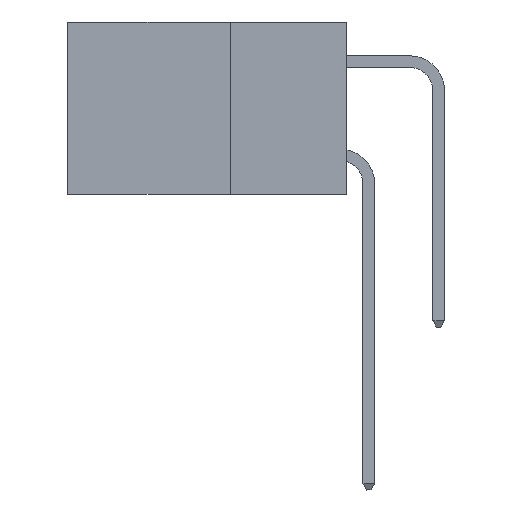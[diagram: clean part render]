
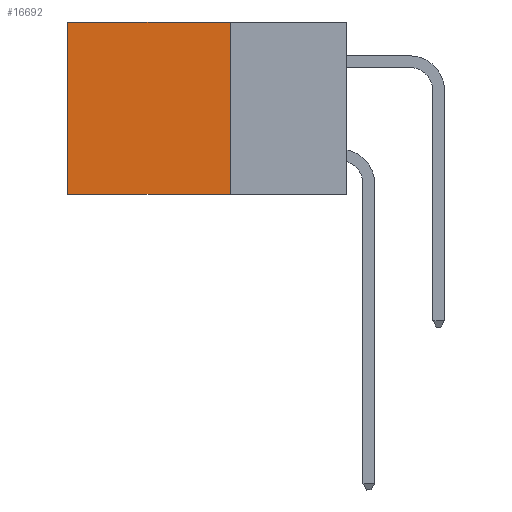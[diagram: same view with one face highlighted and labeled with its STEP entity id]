
A CAD part, left-side view. The second image highlights one B-rep face of the part: STEP entity #16692.
In plain terms, the highlighted planar face has unit normal (-1, 0, 0).
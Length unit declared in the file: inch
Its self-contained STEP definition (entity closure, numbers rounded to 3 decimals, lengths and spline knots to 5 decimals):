
#27 = LINE ( 'NONE', #17710, #20321 ) ;
#296 = DIRECTION ( 'NONE',  ( 0., 1., 0. ) ) ;
#1397 = DIRECTION ( 'NONE',  ( 1., 0., 0. ) ) ;
#1932 = DIRECTION ( 'NONE',  ( 0., 1., 0. ) ) ;
#1976 = VERTEX_POINT ( 'NONE', #5141 ) ;
#2267 = CARTESIAN_POINT ( 'NONE',  ( 0.2875, 0.6, 0. ) ) ;
#2382 = ORIENTED_EDGE ( 'NONE', *, *, #10163, .T. ) ;
#2730 = EDGE_CURVE ( 'NONE', #20494, #1976, #27, .T. ) ;
#3203 = CARTESIAN_POINT ( 'NONE',  ( 0.2875, 0.6, -0.37 ) ) ;
#3978 = EDGE_CURVE ( 'NONE', #20494, #5304, #15951, .T. ) ;
#4183 = CARTESIAN_POINT ( 'NONE',  ( 0.2875, 0.25, 0. ) ) ;
#5141 = CARTESIAN_POINT ( 'NONE',  ( 0.2875, 0.6, 0. ) ) ;
#5304 = VERTEX_POINT ( 'NONE', #8259 ) ;
#5743 = FACE_OUTER_BOUND ( 'NONE', #12007, .T. ) ;
#5843 = DIRECTION ( 'NONE',  ( 0., 0., -1. ) ) ;
#7091 = EDGE_CURVE ( 'NONE', #5304, #24852, #16056, .T. ) ;
#8259 = CARTESIAN_POINT ( 'NONE',  ( 0.2875, 0.25, -0.37 ) ) ;
#8890 = VECTOR ( 'NONE', #16130, 39.37008 ) ;
#9052 = CARTESIAN_POINT ( 'NONE',  ( 0.2875, 0.25, 0. ) ) ;
#10163 = EDGE_CURVE ( 'NONE', #1976, #24852, #10342, .T. ) ;
#10342 = LINE ( 'NONE', #2267, #18902 ) ;
#12007 = EDGE_LOOP ( 'NONE', ( #2382, #25248, #13574, #16932 ) ) ;
#12174 = CARTESIAN_POINT ( 'NONE',  ( 0.2875, 0.25, 0. ) ) ;
#13266 = VECTOR ( 'NONE', #296, 39.37008 ) ;
#13574 = ORIENTED_EDGE ( 'NONE', *, *, #3978, .F. ) ;
#15003 = AXIS2_PLACEMENT_3D ( 'NONE', #9052, #1397, #22782 ) ;
#15951 = LINE ( 'NONE', #4183, #8890 ) ;
#16056 = LINE ( 'NONE', #17455, #13266 ) ;
#16130 = DIRECTION ( 'NONE',  ( 0., 0., -1. ) ) ;
#16692 = ADVANCED_FACE ( 'NONE', ( #5743 ), #19226, .F. ) ;
#16932 = ORIENTED_EDGE ( 'NONE', *, *, #2730, .T. ) ;
#17455 = CARTESIAN_POINT ( 'NONE',  ( 0.2875, 0.25, -0.37 ) ) ;
#17710 = CARTESIAN_POINT ( 'NONE',  ( 0.2875, 0.25, 0. ) ) ;
#18902 = VECTOR ( 'NONE', #5843, 39.37008 ) ;
#19226 = PLANE ( 'NONE',  #15003 ) ;
#20321 = VECTOR ( 'NONE', #1932, 39.37008 ) ;
#20494 = VERTEX_POINT ( 'NONE', #12174 ) ;
#22782 = DIRECTION ( 'NONE',  ( 0., 0., -1. ) ) ;
#24852 = VERTEX_POINT ( 'NONE', #3203 ) ;
#25248 = ORIENTED_EDGE ( 'NONE', *, *, #7091, .F. ) ;
